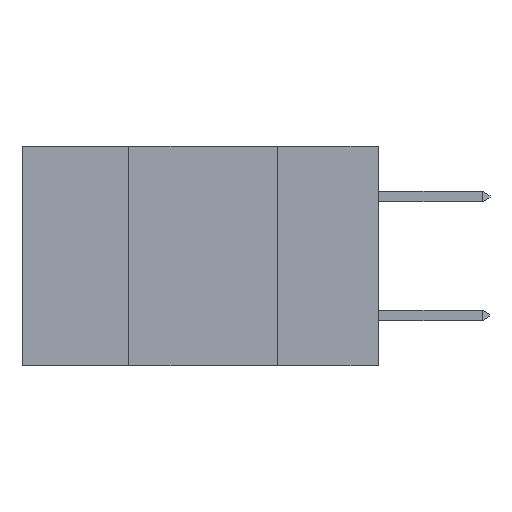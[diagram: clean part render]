
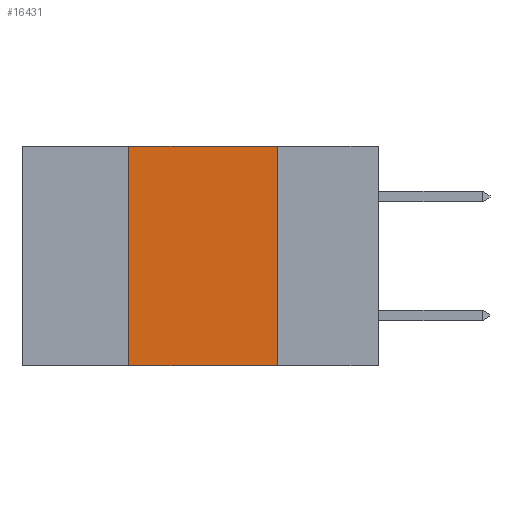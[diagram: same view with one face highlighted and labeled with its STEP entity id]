
A CAD part, left-side view. The second image highlights one B-rep face of the part: STEP entity #16431.
In plain terms, the highlighted planar face has unit normal (-1, 0, 0).
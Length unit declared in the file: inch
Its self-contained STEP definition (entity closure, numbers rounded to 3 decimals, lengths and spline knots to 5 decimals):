
#469 = VECTOR ( 'NONE', #7683, 39.37008 ) ;
#1149 = ORIENTED_EDGE ( 'NONE', *, *, #19350, .F. ) ;
#2114 = LINE ( 'NONE', #28767, #27229 ) ;
#3574 = EDGE_CURVE ( 'NONE', #9413, #19421, #7039, .T. ) ;
#5206 = FACE_OUTER_BOUND ( 'NONE', #8689, .T. ) ;
#5498 = VECTOR ( 'NONE', #19377, 39.37008 ) ;
#5894 = LINE ( 'NONE', #30840, #18019 ) ;
#7039 = LINE ( 'NONE', #28272, #469 ) ;
#7683 = DIRECTION ( 'NONE',  ( 0., 0., -1. ) ) ;
#7954 = CARTESIAN_POINT ( 'NONE',  ( 0., 0.42, -0.37 ) ) ;
#8689 = EDGE_LOOP ( 'NONE', ( #24785, #1149, #21385, #22897 ) ) ;
#9413 = VERTEX_POINT ( 'NONE', #11997 ) ;
#9585 = CARTESIAN_POINT ( 'NONE',  ( 0., 0.6, 0. ) ) ;
#9794 = CARTESIAN_POINT ( 'NONE',  ( 0., 0.17, -0.37 ) ) ;
#11411 = DIRECTION ( 'NONE',  ( 0., -1., 0. ) ) ;
#11941 = LINE ( 'NONE', #9585, #5498 ) ;
#11997 = CARTESIAN_POINT ( 'NONE',  ( 0., 0.17, 0. ) ) ;
#12066 = CARTESIAN_POINT ( 'NONE',  ( 0., 0.6, 0. ) ) ;
#12161 = CARTESIAN_POINT ( 'NONE',  ( 0., 0.42, 0. ) ) ;
#12170 = DIRECTION ( 'NONE',  ( 1., 0., 0. ) ) ;
#12554 = VERTEX_POINT ( 'NONE', #7954 ) ;
#13033 = VERTEX_POINT ( 'NONE', #12161 ) ;
#16431 = ADVANCED_FACE ( 'NONE', ( #5206 ), #26744, .F. ) ;
#16651 = DIRECTION ( 'NONE',  ( 0., 0., 1. ) ) ;
#18019 = VECTOR ( 'NONE', #11411, 39.37008 ) ;
#19151 = EDGE_CURVE ( 'NONE', #12554, #19421, #5894, .T. ) ;
#19350 = EDGE_CURVE ( 'NONE', #13033, #9413, #11941, .T. ) ;
#19377 = DIRECTION ( 'NONE',  ( 0., -1., 0. ) ) ;
#19421 = VERTEX_POINT ( 'NONE', #9794 ) ;
#20243 = AXIS2_PLACEMENT_3D ( 'NONE', #12066, #12170, #29164 ) ;
#21385 = ORIENTED_EDGE ( 'NONE', *, *, #26983, .F. ) ;
#22897 = ORIENTED_EDGE ( 'NONE', *, *, #19151, .T. ) ;
#24785 = ORIENTED_EDGE ( 'NONE', *, *, #3574, .F. ) ;
#26744 = PLANE ( 'NONE',  #20243 ) ;
#26983 = EDGE_CURVE ( 'NONE', #12554, #13033, #2114, .T. ) ;
#27229 = VECTOR ( 'NONE', #16651, 39.37008 ) ;
#28272 = CARTESIAN_POINT ( 'NONE',  ( 0., 0.17, 0. ) ) ;
#28767 = CARTESIAN_POINT ( 'NONE',  ( 0., 0.42, 0. ) ) ;
#29164 = DIRECTION ( 'NONE',  ( 0., 0., -1. ) ) ;
#30840 = CARTESIAN_POINT ( 'NONE',  ( 0., 0.6, -0.37 ) ) ;
